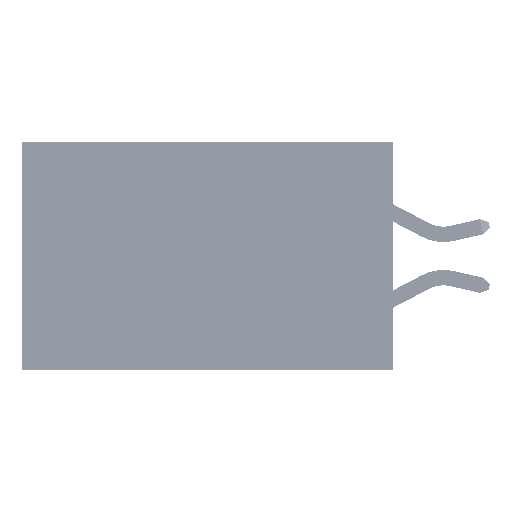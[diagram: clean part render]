
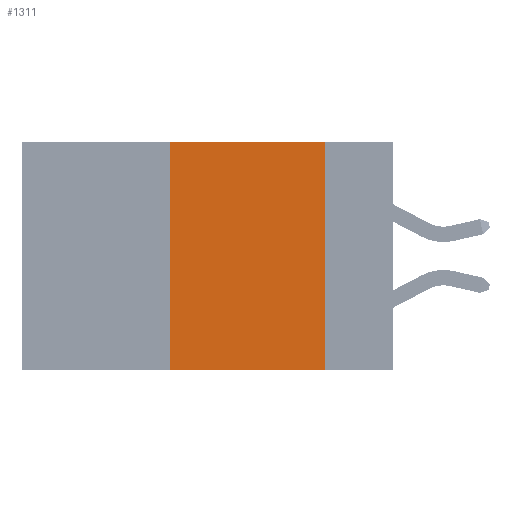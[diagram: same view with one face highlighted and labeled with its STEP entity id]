
A CAD part, left-side view. The second image highlights one B-rep face of the part: STEP entity #1311.
In plain terms, the highlighted planar face has unit normal (-1, 0, 0).
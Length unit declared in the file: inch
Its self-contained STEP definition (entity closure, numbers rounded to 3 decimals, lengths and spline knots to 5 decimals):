
#35 = EDGE_CURVE ( 'NONE', #25090, #9510, #19097, .T. ) ;
#1311 = ADVANCED_FACE ( 'NONE', ( #27812 ), #32906, .F. ) ;
#3571 = VECTOR ( 'NONE', #34309, 39.37008 ) ;
#7060 = VECTOR ( 'NONE', #34661, 39.37008 ) ;
#7324 = VERTEX_POINT ( 'NONE', #18949 ) ;
#7570 = CARTESIAN_POINT ( 'NONE',  ( 0., 0.36, 0. ) ) ;
#9104 = VECTOR ( 'NONE', #25588, 39.37008 ) ;
#9471 = VECTOR ( 'NONE', #18009, 39.37008 ) ;
#9510 = VERTEX_POINT ( 'NONE', #28480 ) ;
#9767 = CARTESIAN_POINT ( 'NONE',  ( 0., 0.6, 0. ) ) ;
#13217 = ORIENTED_EDGE ( 'NONE', *, *, #15185, .F. ) ;
#13539 = EDGE_CURVE ( 'NONE', #24134, #25090, #43625, .T. ) ;
#15185 = EDGE_CURVE ( 'NONE', #7324, #24134, #20968, .T. ) ;
#15944 = EDGE_CURVE ( 'NONE', #7324, #9510, #31986, .T. ) ;
#15986 = CARTESIAN_POINT ( 'NONE',  ( 0., 0.11, 0. ) ) ;
#17293 = CARTESIAN_POINT ( 'NONE',  ( 0., 0.11, 0. ) ) ;
#18009 = DIRECTION ( 'NONE',  ( 0., 0., -1. ) ) ;
#18949 = CARTESIAN_POINT ( 'NONE',  ( 0., 0.36, -0.37 ) ) ;
#19097 = LINE ( 'NONE', #17293, #9471 ) ;
#20968 = LINE ( 'NONE', #7570, #9104 ) ;
#21088 = EDGE_LOOP ( 'NONE', ( #28712, #26334, #13217, #31090 ) ) ;
#24134 = VERTEX_POINT ( 'NONE', #42555 ) ;
#25090 = VERTEX_POINT ( 'NONE', #15986 ) ;
#25588 = DIRECTION ( 'NONE',  ( 0., 0., 1. ) ) ;
#26334 = ORIENTED_EDGE ( 'NONE', *, *, #13539, .F. ) ;
#27812 = FACE_OUTER_BOUND ( 'NONE', #21088, .T. ) ;
#28480 = CARTESIAN_POINT ( 'NONE',  ( 0., 0.11, -0.37 ) ) ;
#28712 = ORIENTED_EDGE ( 'NONE', *, *, #35, .F. ) ;
#30753 = AXIS2_PLACEMENT_3D ( 'NONE', #32403, #42375, #42472 ) ;
#30775 = CARTESIAN_POINT ( 'NONE',  ( 0., 0.6, -0.37 ) ) ;
#31090 = ORIENTED_EDGE ( 'NONE', *, *, #15944, .T. ) ;
#31986 = LINE ( 'NONE', #30775, #3571 ) ;
#32403 = CARTESIAN_POINT ( 'NONE',  ( 0., 0.6, 0. ) ) ;
#32906 = PLANE ( 'NONE',  #30753 ) ;
#34309 = DIRECTION ( 'NONE',  ( 0., -1., 0. ) ) ;
#34661 = DIRECTION ( 'NONE',  ( 0., -1., 0. ) ) ;
#42375 = DIRECTION ( 'NONE',  ( 1., 0., 0. ) ) ;
#42472 = DIRECTION ( 'NONE',  ( 0., 0., -1. ) ) ;
#42555 = CARTESIAN_POINT ( 'NONE',  ( 0., 0.36, 0. ) ) ;
#43625 = LINE ( 'NONE', #9767, #7060 ) ;
